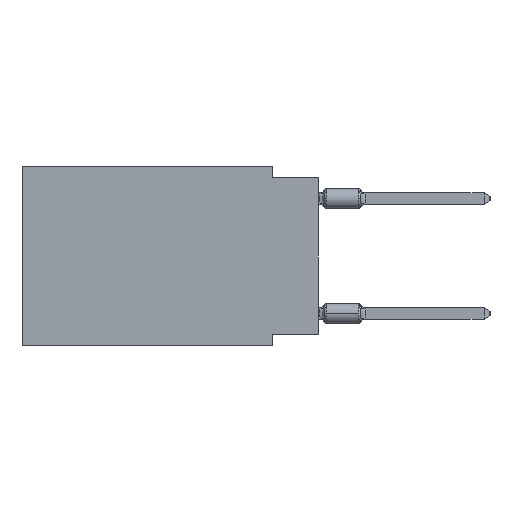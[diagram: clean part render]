
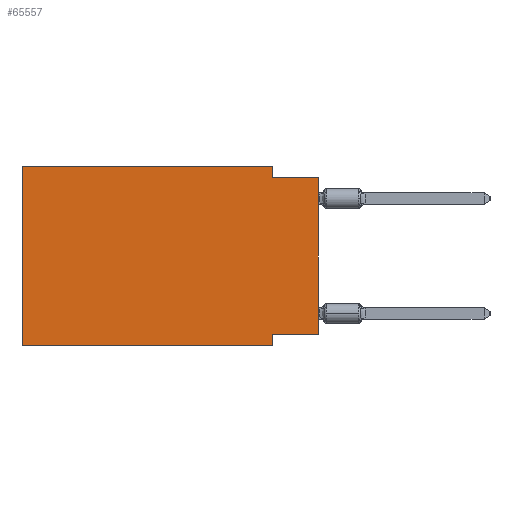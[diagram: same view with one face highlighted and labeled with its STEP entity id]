
A CAD part, left-side view. The second image highlights one B-rep face of the part: STEP entity #65557.
In plain terms, the highlighted planar face has unit normal (-1, 0, 0).
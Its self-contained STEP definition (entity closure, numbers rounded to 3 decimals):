
#849 = CARTESIAN_POINT ( 'NONE',  ( 0., 0., -0.635 ) ) ;
#4508 = ORIENTED_EDGE ( 'NONE', *, *, #50671, .T. ) ;
#5965 = EDGE_LOOP ( 'NONE', ( #41633, #14383, #13626, #31634, #38173, #4508, #59705, #29878 ) ) ;
#6284 = DIRECTION ( 'NONE',  ( 0., 0., 1. ) ) ;
#6327 = CARTESIAN_POINT ( 'NONE',  ( 0., 2.54, -9.906 ) ) ;
#9036 = CARTESIAN_POINT ( 'NONE',  ( 0., 2.54, -9.906 ) ) ;
#10825 = VECTOR ( 'NONE', #28503, 1000. ) ;
#12431 = CARTESIAN_POINT ( 'NONE',  ( 0., 16.383, 0. ) ) ;
#12630 = CARTESIAN_POINT ( 'NONE',  ( 0., 2.54, 0. ) ) ;
#13433 = DIRECTION ( 'NONE',  ( 1., 0., 0. ) ) ;
#13626 = ORIENTED_EDGE ( 'NONE', *, *, #13957, .F. ) ;
#13676 = DIRECTION ( 'NONE',  ( 0., -1., 0. ) ) ;
#13957 = EDGE_CURVE ( 'NONE', #25686, #45910, #22705, .T. ) ;
#14383 = ORIENTED_EDGE ( 'NONE', *, *, #25075, .F. ) ;
#14598 = DIRECTION ( 'NONE',  ( 0., -1., 0. ) ) ;
#15269 = LINE ( 'NONE', #36122, #50321 ) ;
#15654 = LINE ( 'NONE', #62836, #66124 ) ;
#15831 = DIRECTION ( 'NONE',  ( 0., -1., 0. ) ) ;
#16299 = VERTEX_POINT ( 'NONE', #51610 ) ;
#16625 = VERTEX_POINT ( 'NONE', #26809 ) ;
#16832 = CARTESIAN_POINT ( 'NONE',  ( 0., 0., -0.635 ) ) ;
#22705 = LINE ( 'NONE', #43578, #10825 ) ;
#22907 = LINE ( 'NONE', #33517, #62745 ) ;
#23126 = EDGE_CURVE ( 'NONE', #16625, #27792, #24419, .T. ) ;
#24419 = LINE ( 'NONE', #9036, #50984 ) ;
#24975 = VECTOR ( 'NONE', #15831, 1000. ) ;
#25075 = EDGE_CURVE ( 'NONE', #45910, #39195, #36680, .T. ) ;
#25686 = VERTEX_POINT ( 'NONE', #12630 ) ;
#26809 = CARTESIAN_POINT ( 'NONE',  ( 0., 2.54, -9.271 ) ) ;
#27792 = VERTEX_POINT ( 'NONE', #6327 ) ;
#28503 = DIRECTION ( 'NONE',  ( 0., 0., -1. ) ) ;
#29481 = FACE_OUTER_BOUND ( 'NONE', #5965, .T. ) ;
#29878 = ORIENTED_EDGE ( 'NONE', *, *, #32530, .F. ) ;
#30650 = CARTESIAN_POINT ( 'NONE',  ( 0., 0., -9.271 ) ) ;
#31634 = ORIENTED_EDGE ( 'NONE', *, *, #58675, .F. ) ;
#32530 = EDGE_CURVE ( 'NONE', #43167, #16625, #46063, .T. ) ;
#33282 = DIRECTION ( 'NONE',  ( 0., 0., -1. ) ) ;
#33517 = CARTESIAN_POINT ( 'NONE',  ( 0., 16.383, 0. ) ) ;
#35019 = EDGE_CURVE ( 'NONE', #51045, #16299, #15654, .T. ) ;
#36122 = CARTESIAN_POINT ( 'NONE',  ( 0., 16.383, -9.906 ) ) ;
#36680 = LINE ( 'NONE', #16832, #24975 ) ;
#36810 = EDGE_CURVE ( 'NONE', #43167, #39195, #49631, .T. ) ;
#38173 = ORIENTED_EDGE ( 'NONE', *, *, #35019, .F. ) ;
#39195 = VERTEX_POINT ( 'NONE', #849 ) ;
#40005 = VECTOR ( 'NONE', #6284, 1000. ) ;
#41633 = ORIENTED_EDGE ( 'NONE', *, *, #36810, .T. ) ;
#41744 = AXIS2_PLACEMENT_3D ( 'NONE', #12431, #13433, #33282 ) ;
#43167 = VERTEX_POINT ( 'NONE', #56040 ) ;
#43539 = PLANE ( 'NONE',  #41744 ) ;
#43578 = CARTESIAN_POINT ( 'NONE',  ( 0., 2.54, 0. ) ) ;
#45738 = DIRECTION ( 'NONE',  ( 0., 1., 0. ) ) ;
#45910 = VERTEX_POINT ( 'NONE', #45983 ) ;
#45983 = CARTESIAN_POINT ( 'NONE',  ( 0., 2.54, -0.635 ) ) ;
#46063 = LINE ( 'NONE', #30650, #47145 ) ;
#46776 = DIRECTION ( 'NONE',  ( 0., 0., 1. ) ) ;
#47145 = VECTOR ( 'NONE', #45738, 1000. ) ;
#49631 = LINE ( 'NONE', #53146, #40005 ) ;
#50321 = VECTOR ( 'NONE', #14598, 1000. ) ;
#50671 = EDGE_CURVE ( 'NONE', #51045, #27792, #15269, .T. ) ;
#50984 = VECTOR ( 'NONE', #54882, 1000. ) ;
#51045 = VERTEX_POINT ( 'NONE', #57852 ) ;
#51610 = CARTESIAN_POINT ( 'NONE',  ( 0., 16.383, 0. ) ) ;
#53146 = CARTESIAN_POINT ( 'NONE',  ( 0., 0., 0. ) ) ;
#54882 = DIRECTION ( 'NONE',  ( 0., 0., -1. ) ) ;
#56040 = CARTESIAN_POINT ( 'NONE',  ( 0., 0., -9.271 ) ) ;
#57852 = CARTESIAN_POINT ( 'NONE',  ( 0., 16.383, -9.906 ) ) ;
#58675 = EDGE_CURVE ( 'NONE', #16299, #25686, #22907, .T. ) ;
#59705 = ORIENTED_EDGE ( 'NONE', *, *, #23126, .F. ) ;
#62745 = VECTOR ( 'NONE', #13676, 1000. ) ;
#62836 = CARTESIAN_POINT ( 'NONE',  ( 0., 16.383, 0. ) ) ;
#65557 = ADVANCED_FACE ( 'NONE', ( #29481 ), #43539, .F. ) ;
#66124 = VECTOR ( 'NONE', #46776, 1000. ) ;
